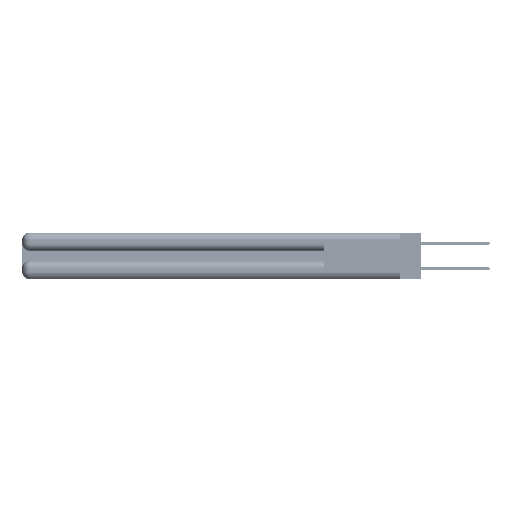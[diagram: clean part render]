
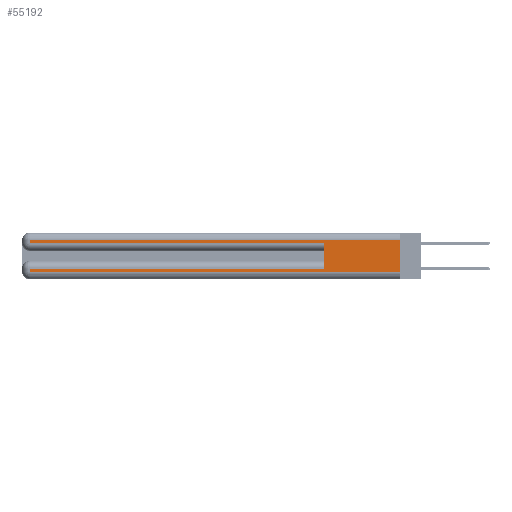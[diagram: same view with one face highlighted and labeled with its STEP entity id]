
A CAD part, left-side view. The second image highlights one B-rep face of the part: STEP entity #55192.
In plain terms, the highlighted planar face has unit normal (-1, 0, 0).
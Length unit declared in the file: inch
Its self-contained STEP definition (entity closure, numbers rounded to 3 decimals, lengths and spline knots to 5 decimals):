
#1730 = DIRECTION ( 'NONE',  ( 0., -1., 0. ) ) ;
#1814 = DIRECTION ( 'NONE',  ( 0., 0., -1. ) ) ;
#2556 = ORIENTED_EDGE ( 'NONE', *, *, #18854, .F. ) ;
#3045 = CARTESIAN_POINT ( 'NONE',  ( 0., 0., 0.31 ) ) ;
#3334 = EDGE_CURVE ( 'NONE', #33691, #4321, #51682, .T. ) ;
#3812 = LINE ( 'NONE', #37078, #8624 ) ;
#4321 = VERTEX_POINT ( 'NONE', #5103 ) ;
#5103 = CARTESIAN_POINT ( 'NONE',  ( 0., 2.94, 0.06 ) ) ;
#5203 = DIRECTION ( 'NONE',  ( 0., 0., -1. ) ) ;
#5226 = VERTEX_POINT ( 'NONE', #20394 ) ;
#5432 = VERTEX_POINT ( 'NONE', #26521 ) ;
#5540 = ORIENTED_EDGE ( 'NONE', *, *, #27713, .T. ) ;
#5698 = VECTOR ( 'NONE', #17543, 39.37008 ) ;
#5915 = LINE ( 'NONE', #50282, #52240 ) ;
#8048 = ORIENTED_EDGE ( 'NONE', *, *, #42674, .T. ) ;
#8624 = VECTOR ( 'NONE', #18493, 39.37008 ) ;
#9450 = PLANE ( 'NONE',  #34326 ) ;
#11881 = LINE ( 'NONE', #35528, #5698 ) ;
#12645 = EDGE_CURVE ( 'NONE', #54202, #44426, #5915, .T. ) ;
#13346 = DIRECTION ( 'NONE',  ( 0., 0., -1. ) ) ;
#17543 = DIRECTION ( 'NONE',  ( 0., -1., 0. ) ) ;
#18493 = DIRECTION ( 'NONE',  ( 0., 0., -1. ) ) ;
#18854 = EDGE_CURVE ( 'NONE', #5432, #28520, #3812, .T. ) ;
#20276 = DIRECTION ( 'NONE',  ( 0., 1., 0. ) ) ;
#20280 = VECTOR ( 'NONE', #29631, 39.37008 ) ;
#20394 = CARTESIAN_POINT ( 'NONE',  ( 0., 0.6, 0.285 ) ) ;
#20549 = DIRECTION ( 'NONE',  ( 0., 0., 1. ) ) ;
#24299 = ORIENTED_EDGE ( 'NONE', *, *, #48948, .T. ) ;
#24667 = VECTOR ( 'NONE', #1730, 39.37008 ) ;
#25244 = LINE ( 'NONE', #55292, #47427 ) ;
#26521 = CARTESIAN_POINT ( 'NONE',  ( 0., 0., 0.31 ) ) ;
#26857 = VERTEX_POINT ( 'NONE', #40515 ) ;
#27338 = CARTESIAN_POINT ( 'NONE',  ( 0., 0., 0.37 ) ) ;
#27713 = EDGE_CURVE ( 'NONE', #26857, #33691, #25244, .T. ) ;
#28520 = VERTEX_POINT ( 'NONE', #43254 ) ;
#28802 = VECTOR ( 'NONE', #20549, 39.37008 ) ;
#28985 = CARTESIAN_POINT ( 'NONE',  ( 0., 2.94, 0.31 ) ) ;
#29631 = DIRECTION ( 'NONE',  ( 0., 1., 0. ) ) ;
#30929 = EDGE_CURVE ( 'NONE', #26857, #5226, #47534, .T. ) ;
#30933 = CARTESIAN_POINT ( 'NONE',  ( 0., 2.94, 0.285 ) ) ;
#31797 = DIRECTION ( 'NONE',  ( 1., 0., 0. ) ) ;
#31870 = EDGE_CURVE ( 'NONE', #4321, #28520, #11881, .T. ) ;
#33691 = VERTEX_POINT ( 'NONE', #51829 ) ;
#34326 = AXIS2_PLACEMENT_3D ( 'NONE', #27338, #31797, #5203 ) ;
#34920 = ORIENTED_EDGE ( 'NONE', *, *, #30929, .F. ) ;
#35528 = CARTESIAN_POINT ( 'NONE',  ( 0., 0., 0.06 ) ) ;
#36476 = VECTOR ( 'NONE', #13346, 39.37008 ) ;
#37078 = CARTESIAN_POINT ( 'NONE',  ( 0., 0., 0.37 ) ) ;
#38485 = FACE_OUTER_BOUND ( 'NONE', #50175, .T. ) ;
#40515 = CARTESIAN_POINT ( 'NONE',  ( 0., 0.6, 0.085 ) ) ;
#42674 = EDGE_CURVE ( 'NONE', #44426, #5226, #56532, .T. ) ;
#43254 = CARTESIAN_POINT ( 'NONE',  ( 0., 0., 0.06 ) ) ;
#44426 = VERTEX_POINT ( 'NONE', #30933 ) ;
#44499 = LINE ( 'NONE', #3045, #20280 ) ;
#47064 = CARTESIAN_POINT ( 'NONE',  ( 0., 0.6, 0.145 ) ) ;
#47427 = VECTOR ( 'NONE', #20276, 39.37008 ) ;
#47534 = LINE ( 'NONE', #47064, #28802 ) ;
#48948 = EDGE_CURVE ( 'NONE', #5432, #54202, #44499, .T. ) ;
#49109 = CARTESIAN_POINT ( 'NONE',  ( 0., 2.94, 0.37 ) ) ;
#50175 = EDGE_LOOP ( 'NONE', ( #2556, #24299, #57051, #8048, #34920, #5540, #52825, #51715 ) ) ;
#50282 = CARTESIAN_POINT ( 'NONE',  ( 0., 2.94, 0.37 ) ) ;
#51682 = LINE ( 'NONE', #49109, #36476 ) ;
#51715 = ORIENTED_EDGE ( 'NONE', *, *, #31870, .T. ) ;
#51829 = CARTESIAN_POINT ( 'NONE',  ( 0., 2.94, 0.085 ) ) ;
#52240 = VECTOR ( 'NONE', #1814, 39.37008 ) ;
#52825 = ORIENTED_EDGE ( 'NONE', *, *, #3334, .T. ) ;
#54202 = VERTEX_POINT ( 'NONE', #28985 ) ;
#54621 = CARTESIAN_POINT ( 'NONE',  ( 0., 0., 0.285 ) ) ;
#55192 = ADVANCED_FACE ( 'NONE', ( #38485 ), #9450, .F. ) ;
#55292 = CARTESIAN_POINT ( 'NONE',  ( 0., 0., 0.085 ) ) ;
#56532 = LINE ( 'NONE', #54621, #24667 ) ;
#57051 = ORIENTED_EDGE ( 'NONE', *, *, #12645, .T. ) ;
